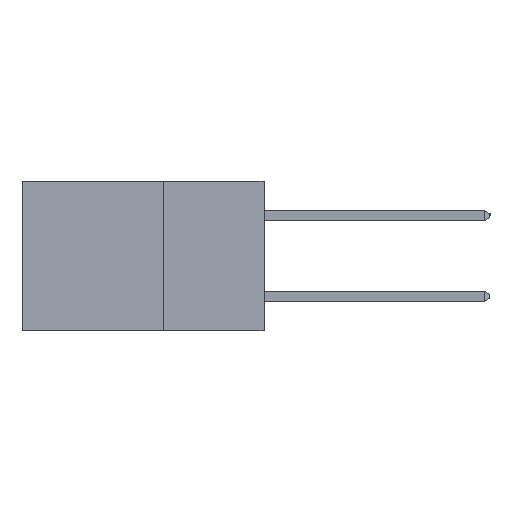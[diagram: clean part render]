
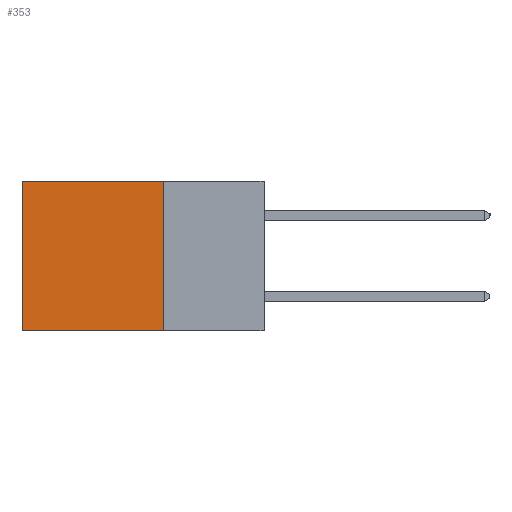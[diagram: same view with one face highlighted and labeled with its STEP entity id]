
A CAD part, left-side view. The second image highlights one B-rep face of the part: STEP entity #353.
In plain terms, the highlighted planar face has unit normal (-1, 0, 0).
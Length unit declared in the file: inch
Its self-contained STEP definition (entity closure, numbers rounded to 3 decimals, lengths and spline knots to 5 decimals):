
#353 = ADVANCED_FACE ( 'NONE', ( #14116 ), #8483, .F. ) ;
#383 = VECTOR ( 'NONE', #22188, 39.37008 ) ;
#832 = ORIENTED_EDGE ( 'NONE', *, *, #11308, .F. ) ;
#1610 = ORIENTED_EDGE ( 'NONE', *, *, #3190, .T. ) ;
#2073 = LINE ( 'NONE', #2315, #12808 ) ;
#2315 = CARTESIAN_POINT ( 'NONE',  ( 0.2615, 0.6, -0.37 ) ) ;
#3190 = EDGE_CURVE ( 'NONE', #19058, #13874, #2073, .T. ) ;
#3537 = VERTEX_POINT ( 'NONE', #22269 ) ;
#3584 = DIRECTION ( 'NONE',  ( 0., 1., 0. ) ) ;
#4598 = DIRECTION ( 'NONE',  ( 0., 0., -1. ) ) ;
#4609 = VERTEX_POINT ( 'NONE', #13734 ) ;
#6722 = DIRECTION ( 'NONE',  ( 1., 0., 0. ) ) ;
#8483 = PLANE ( 'NONE',  #12657 ) ;
#9220 = CARTESIAN_POINT ( 'NONE',  ( 0.2615, 0.25, -0.37 ) ) ;
#9694 = EDGE_CURVE ( 'NONE', #4609, #19058, #10992, .T. ) ;
#10321 = VECTOR ( 'NONE', #3584, 39.37008 ) ;
#10992 = LINE ( 'NONE', #20323, #10321 ) ;
#11308 = EDGE_CURVE ( 'NONE', #4609, #3537, #16488, .T. ) ;
#11573 = DIRECTION ( 'NONE',  ( 0., 0., -1. ) ) ;
#12657 = AXIS2_PLACEMENT_3D ( 'NONE', #21690, #6722, #4598 ) ;
#12808 = VECTOR ( 'NONE', #11573, 39.37008 ) ;
#12906 = ORIENTED_EDGE ( 'NONE', *, *, #19390, .F. ) ;
#13017 = CARTESIAN_POINT ( 'NONE',  ( 0.2615, 0.6, 0. ) ) ;
#13235 = DIRECTION ( 'NONE',  ( 0., 1., 0. ) ) ;
#13734 = CARTESIAN_POINT ( 'NONE',  ( 0.2615, 0.25, 0. ) ) ;
#13874 = VERTEX_POINT ( 'NONE', #21338 ) ;
#14116 = FACE_OUTER_BOUND ( 'NONE', #20439, .T. ) ;
#16488 = LINE ( 'NONE', #21944, #383 ) ;
#19058 = VERTEX_POINT ( 'NONE', #13017 ) ;
#19390 = EDGE_CURVE ( 'NONE', #3537, #13874, #22435, .T. ) ;
#20323 = CARTESIAN_POINT ( 'NONE',  ( 0.2615, 0.25, 0. ) ) ;
#20439 = EDGE_LOOP ( 'NONE', ( #1610, #12906, #832, #24219 ) ) ;
#21338 = CARTESIAN_POINT ( 'NONE',  ( 0.2615, 0.6, -0.37 ) ) ;
#21690 = CARTESIAN_POINT ( 'NONE',  ( 0.2615, 0.25, -0.37 ) ) ;
#21944 = CARTESIAN_POINT ( 'NONE',  ( 0.2615, 0.25, -0.37 ) ) ;
#22188 = DIRECTION ( 'NONE',  ( 0., 0., -1. ) ) ;
#22269 = CARTESIAN_POINT ( 'NONE',  ( 0.2615, 0.25, -0.37 ) ) ;
#22435 = LINE ( 'NONE', #9220, #22497 ) ;
#22497 = VECTOR ( 'NONE', #13235, 39.37008 ) ;
#24219 = ORIENTED_EDGE ( 'NONE', *, *, #9694, .T. ) ;
